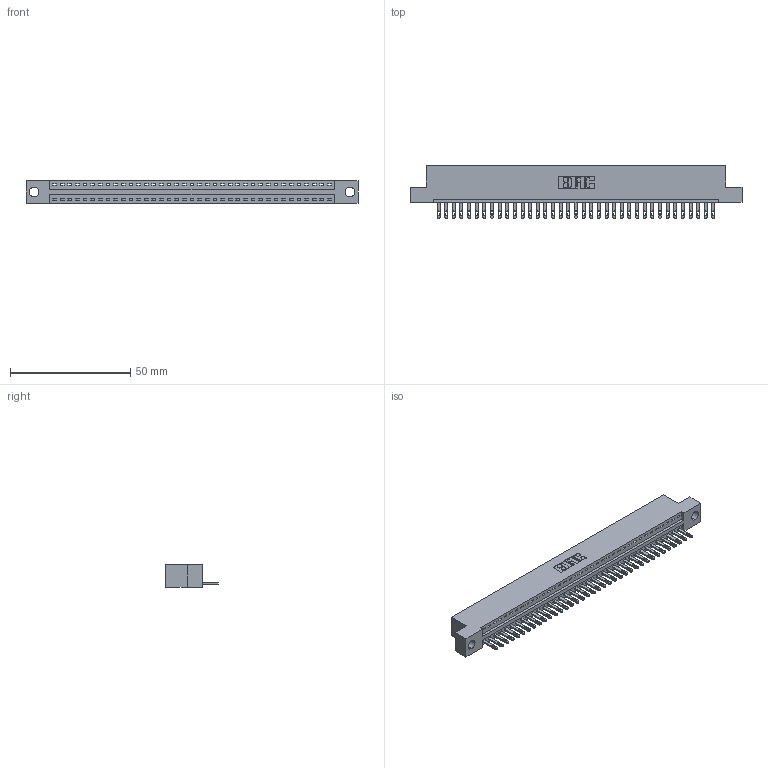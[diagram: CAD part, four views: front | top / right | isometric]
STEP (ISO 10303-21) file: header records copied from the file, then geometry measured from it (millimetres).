
FILE_DESCRIPTION (( 'STEP AP203' ), '1' );
FILE_NAME ('346-037-500-104.STEP', '2022-05-07T01:56:21', ( '' ), ( '' ), 'SwSTEP 2.0', 'SolidWorks 2020', '' );
FILE_SCHEMA (( 'CONFIG_CONTROL_DESIGN' ));
Length unit declared in the file: inch
Products named in the file (3): 345-292-001_345-293-100; 346-037-500-104; 346 Part_Flush Mounting Lugs - 0.156 Dia-TH
Assembly tree (38 placements, depth 2):
  346-037-500-104
    346 Part_Flush Mounting Lugs - 0.156 Dia-TH
    345-292-001_345-293-100  x37
Bounding box: 138.05 x 21.84 x 9.4 mm (x, y, z)
Volume: 13096.8 mm3; surface area: 16238.9 mm2
Topology: 38 solids, 38 shells, 2134 faces, 6581 edges, 4386 vertices
Faces by surface type: plane 1348, cylinder 786
Entity records: 23985 total; most frequent: CARTESIAN_POINT 4121, ORIENTED_EDGE 4090, DIRECTION 3643, EDGE_CURVE 2045, LINE 1761, VECTOR 1761, VERTEX_POINT 1362, AXIS2_PLACEMENT_3D 941
